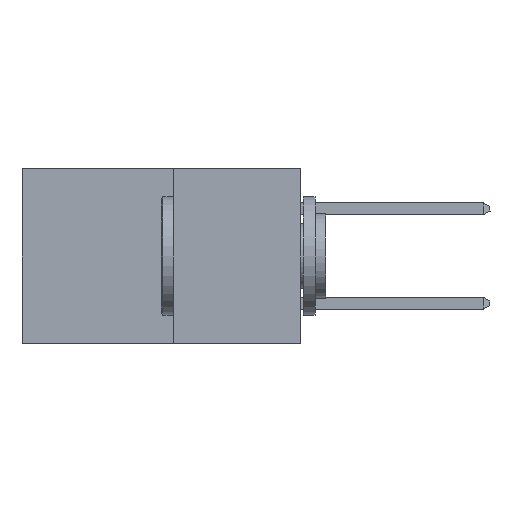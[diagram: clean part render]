
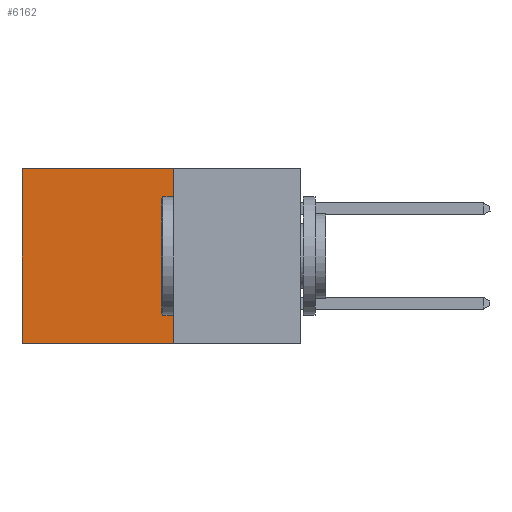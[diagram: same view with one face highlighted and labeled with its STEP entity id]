
A CAD part, left-side view. The second image highlights one B-rep face of the part: STEP entity #6162.
In plain terms, the highlighted planar face has unit normal (-1, 0, 0).
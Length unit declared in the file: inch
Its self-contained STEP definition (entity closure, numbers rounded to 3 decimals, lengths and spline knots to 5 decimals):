
#31 = FACE_OUTER_BOUND ( 'NONE', #27098, .T. ) ;
#245 = VECTOR ( 'NONE', #9367, 39.37008 ) ;
#711 = CARTESIAN_POINT ( 'NONE',  ( 0.277, 0.27, 0. ) ) ;
#1104 = VECTOR ( 'NONE', #14461, 39.37008 ) ;
#1496 = EDGE_CURVE ( 'NONE', #14242, #27511, #21819, .T. ) ;
#3431 = DIRECTION ( 'NONE',  ( 0., 1., 0. ) ) ;
#3688 = CARTESIAN_POINT ( 'NONE',  ( 0.277, 0.27, 0. ) ) ;
#5238 = EDGE_CURVE ( 'NONE', #13497, #10932, #27608, .T. ) ;
#6162 = ADVANCED_FACE ( 'NONE', ( #31 ), #26266, .F. ) ;
#6592 = ORIENTED_EDGE ( 'NONE', *, *, #12983, .F. ) ;
#7174 = CARTESIAN_POINT ( 'NONE',  ( 0.277, 0.59, -0.37 ) ) ;
#9367 = DIRECTION ( 'NONE',  ( 0., 0., -1. ) ) ;
#10932 = VERTEX_POINT ( 'NONE', #25881 ) ;
#12293 = CARTESIAN_POINT ( 'NONE',  ( 0.277, 0.27, -0.37 ) ) ;
#12328 = DIRECTION ( 'NONE',  ( 0., 1., 0. ) ) ;
#12766 = LINE ( 'NONE', #12293, #1104 ) ;
#12875 = CARTESIAN_POINT ( 'NONE',  ( 0.277, 0.27, -0.37 ) ) ;
#12983 = EDGE_CURVE ( 'NONE', #14242, #13497, #12766, .T. ) ;
#13497 = VERTEX_POINT ( 'NONE', #13684 ) ;
#13684 = CARTESIAN_POINT ( 'NONE',  ( 0.277, 0.27, -0.37 ) ) ;
#14242 = VERTEX_POINT ( 'NONE', #711 ) ;
#14461 = DIRECTION ( 'NONE',  ( 0., 0., -1. ) ) ;
#16046 = VECTOR ( 'NONE', #3431, 39.37008 ) ;
#17579 = ORIENTED_EDGE ( 'NONE', *, *, #1496, .T. ) ;
#17718 = LINE ( 'NONE', #7174, #245 ) ;
#18434 = ORIENTED_EDGE ( 'NONE', *, *, #21021, .T. ) ;
#19342 = CARTESIAN_POINT ( 'NONE',  ( 0.277, 0.59, 0. ) ) ;
#21021 = EDGE_CURVE ( 'NONE', #27511, #10932, #17718, .T. ) ;
#21819 = LINE ( 'NONE', #3688, #16046 ) ;
#21971 = VECTOR ( 'NONE', #12328, 39.37008 ) ;
#25881 = CARTESIAN_POINT ( 'NONE',  ( 0.277, 0.59, -0.37 ) ) ;
#26146 = ORIENTED_EDGE ( 'NONE', *, *, #5238, .F. ) ;
#26202 = DIRECTION ( 'NONE',  ( 0., 0., -1. ) ) ;
#26234 = DIRECTION ( 'NONE',  ( 1., 0., 0. ) ) ;
#26259 = CARTESIAN_POINT ( 'NONE',  ( 0.277, 0.27, -0.37 ) ) ;
#26266 = PLANE ( 'NONE',  #27447 ) ;
#27098 = EDGE_LOOP ( 'NONE', ( #18434, #26146, #6592, #17579 ) ) ;
#27447 = AXIS2_PLACEMENT_3D ( 'NONE', #26259, #26234, #26202 ) ;
#27511 = VERTEX_POINT ( 'NONE', #19342 ) ;
#27608 = LINE ( 'NONE', #12875, #21971 ) ;
